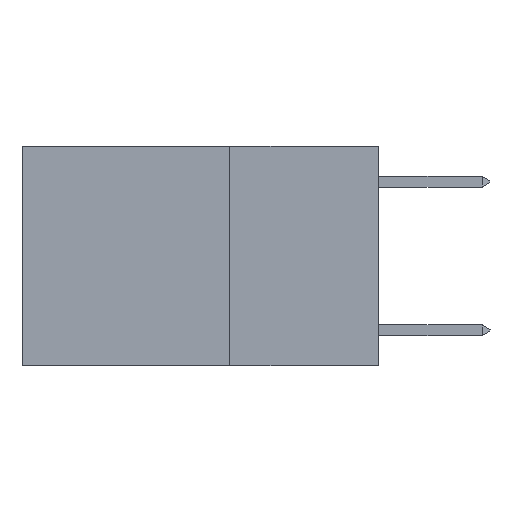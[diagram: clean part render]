
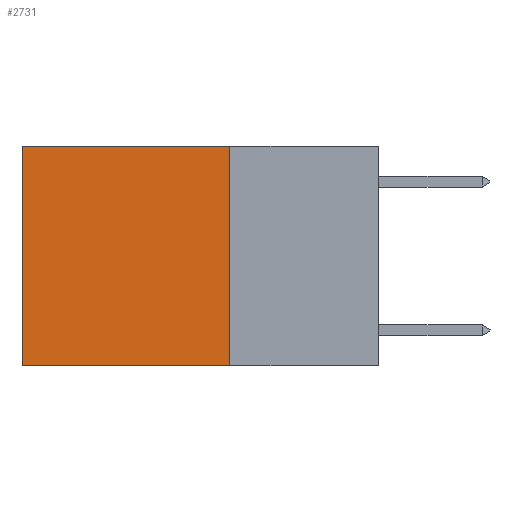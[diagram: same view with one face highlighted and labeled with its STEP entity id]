
A CAD part, left-side view. The second image highlights one B-rep face of the part: STEP entity #2731.
In plain terms, the highlighted planar face has unit normal (-1, 0, 0).
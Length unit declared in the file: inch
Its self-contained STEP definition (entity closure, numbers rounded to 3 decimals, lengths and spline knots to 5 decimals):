
#23 = CARTESIAN_POINT ( 'NONE',  ( 0.2625, 0.6, -0.37 ) ) ;
#360 = EDGE_CURVE ( 'NONE', #15246, #3173, #20263, .T. ) ;
#2731 = ADVANCED_FACE ( 'NONE', ( #5776 ), #9607, .F. ) ;
#2824 = EDGE_CURVE ( 'NONE', #12340, #14140, #5219, .T. ) ;
#3133 = DIRECTION ( 'NONE',  ( 0., 0., -1. ) ) ;
#3173 = VERTEX_POINT ( 'NONE', #14081 ) ;
#3370 = EDGE_LOOP ( 'NONE', ( #8474, #9804, #7544, #6132 ) ) ;
#3746 = EDGE_CURVE ( 'NONE', #3173, #14140, #17705, .T. ) ;
#3874 = CARTESIAN_POINT ( 'NONE',  ( 0.2625, 0.6, 0. ) ) ;
#4334 = DIRECTION ( 'NONE',  ( 0., 1., 0. ) ) ;
#5141 = DIRECTION ( 'NONE',  ( 0., 1., 0. ) ) ;
#5144 = VECTOR ( 'NONE', #5141, 39.37008 ) ;
#5205 = CARTESIAN_POINT ( 'NONE',  ( 0.2625, 0.25, -0.37 ) ) ;
#5219 = LINE ( 'NONE', #5205, #5144 ) ;
#5776 = FACE_OUTER_BOUND ( 'NONE', #3370, .T. ) ;
#6132 = ORIENTED_EDGE ( 'NONE', *, *, #360, .T. ) ;
#6703 = CARTESIAN_POINT ( 'NONE',  ( 0.2625, 0.25, 0. ) ) ;
#7544 = ORIENTED_EDGE ( 'NONE', *, *, #10496, .F. ) ;
#7771 = VECTOR ( 'NONE', #15992, 39.37008 ) ;
#8250 = LINE ( 'NONE', #15954, #7771 ) ;
#8395 = DIRECTION ( 'NONE',  ( 0., 0., -1. ) ) ;
#8474 = ORIENTED_EDGE ( 'NONE', *, *, #3746, .T. ) ;
#8565 = DIRECTION ( 'NONE',  ( 1., 0., 0. ) ) ;
#8981 = CARTESIAN_POINT ( 'NONE',  ( 0.2625, 0.25, 0. ) ) ;
#9607 = PLANE ( 'NONE',  #11953 ) ;
#9804 = ORIENTED_EDGE ( 'NONE', *, *, #2824, .F. ) ;
#10496 = EDGE_CURVE ( 'NONE', #15246, #12340, #8250, .T. ) ;
#10949 = CARTESIAN_POINT ( 'NONE',  ( 0.2625, 0.25, -0.37 ) ) ;
#11953 = AXIS2_PLACEMENT_3D ( 'NONE', #8981, #8565, #8395 ) ;
#12340 = VERTEX_POINT ( 'NONE', #10949 ) ;
#14081 = CARTESIAN_POINT ( 'NONE',  ( 0.2625, 0.6, 0. ) ) ;
#14140 = VERTEX_POINT ( 'NONE', #23 ) ;
#15246 = VERTEX_POINT ( 'NONE', #15582 ) ;
#15582 = CARTESIAN_POINT ( 'NONE',  ( 0.2625, 0.25, 0. ) ) ;
#15954 = CARTESIAN_POINT ( 'NONE',  ( 0.2625, 0.25, 0. ) ) ;
#15992 = DIRECTION ( 'NONE',  ( 0., 0., -1. ) ) ;
#17705 = LINE ( 'NONE', #3874, #18274 ) ;
#18274 = VECTOR ( 'NONE', #3133, 39.37008 ) ;
#19893 = VECTOR ( 'NONE', #4334, 39.37008 ) ;
#20263 = LINE ( 'NONE', #6703, #19893 ) ;
